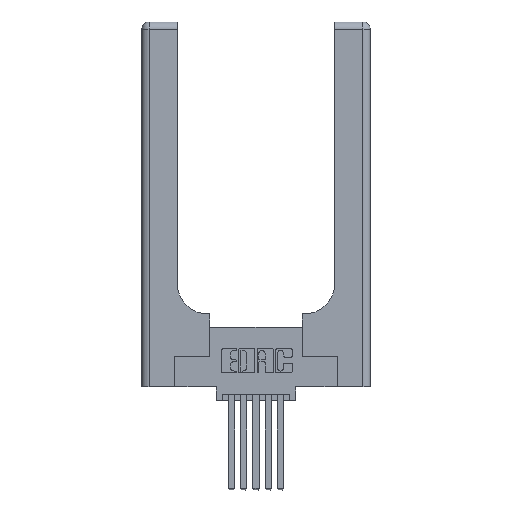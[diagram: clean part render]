
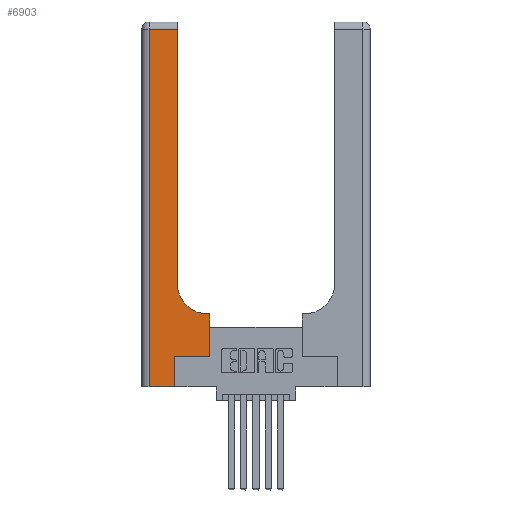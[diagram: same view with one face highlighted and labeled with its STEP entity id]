
A CAD part, top view. The second image highlights one B-rep face of the part: STEP entity #6903.
In plain terms, the highlighted planar face has unit normal (0, 0, 1).
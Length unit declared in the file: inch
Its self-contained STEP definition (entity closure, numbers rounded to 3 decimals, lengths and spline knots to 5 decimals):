
#79 = VERTEX_POINT ( 'NONE', #13041 ) ;
#231 = VECTOR ( 'NONE', #11120, 39.37008 ) ;
#462 = VERTEX_POINT ( 'NONE', #11801 ) ;
#568 = CARTESIAN_POINT ( 'NONE',  ( 0.2915, 3., 0.37 ) ) ;
#622 = LINE ( 'NONE', #8475, #11887 ) ;
#912 = DIRECTION ( 'NONE',  ( 0., 1., 0. ) ) ;
#1087 = VERTEX_POINT ( 'NONE', #9280 ) ;
#1621 = CARTESIAN_POINT ( 'NONE',  ( 0.2915, 0.6, 0.37 ) ) ;
#1825 = ORIENTED_EDGE ( 'NONE', *, *, #13421, .T. ) ;
#1846 = CARTESIAN_POINT ( 'NONE',  ( 0.269, 0.25, 0.37 ) ) ;
#1917 = ORIENTED_EDGE ( 'NONE', *, *, #9651, .T. ) ;
#2306 = VECTOR ( 'NONE', #8315, 39.37008 ) ;
#2355 = CARTESIAN_POINT ( 'NONE',  ( 0., 3., 0.37 ) ) ;
#2364 = VERTEX_POINT ( 'NONE', #2557 ) ;
#2557 = CARTESIAN_POINT ( 'NONE',  ( 0.2915, 2.94, 0.37 ) ) ;
#2765 = DIRECTION ( 'NONE',  ( -1., 0., 0. ) ) ;
#2800 = EDGE_CURVE ( 'NONE', #8301, #1087, #9077, .T. ) ;
#2803 = LINE ( 'NONE', #1846, #5424 ) ;
#2892 = ORIENTED_EDGE ( 'NONE', *, *, #10429, .T. ) ;
#2971 = AXIS2_PLACEMENT_3D ( 'NONE', #6559, #13859, #7617 ) ;
#3492 = EDGE_CURVE ( 'NONE', #11928, #79, #4514, .T. ) ;
#3666 = VERTEX_POINT ( 'NONE', #7474 ) ;
#3703 = VERTEX_POINT ( 'NONE', #7651 ) ;
#3852 = EDGE_CURVE ( 'NONE', #2364, #3666, #8396, .T. ) ;
#4004 = CARTESIAN_POINT ( 'NONE',  ( 0.5585, 0.25, 0.37 ) ) ;
#4514 = LINE ( 'NONE', #10444, #10226 ) ;
#5068 = LINE ( 'NONE', #1621, #7611 ) ;
#5331 = VECTOR ( 'NONE', #912, 39.37008 ) ;
#5424 = VECTOR ( 'NONE', #6294, 39.37008 ) ;
#5729 = DIRECTION ( 'NONE',  ( 0., 0., -1. ) ) ;
#6140 = ORIENTED_EDGE ( 'NONE', *, *, #2800, .T. ) ;
#6294 = DIRECTION ( 'NONE',  ( 1., 0., 0. ) ) ;
#6405 = DIRECTION ( 'NONE',  ( 0., -1., 0. ) ) ;
#6559 = CARTESIAN_POINT ( 'NONE',  ( 0.5415, 0.85, 0.37 ) ) ;
#6763 = AXIS2_PLACEMENT_3D ( 'NONE', #2355, #5729, #13114 ) ;
#6903 = ADVANCED_FACE ( 'NONE', ( #11786 ), #12082, .F. ) ;
#7474 = CARTESIAN_POINT ( 'NONE',  ( 0.06, 2.94, 0.37 ) ) ;
#7580 = CARTESIAN_POINT ( 'NONE',  ( 0.269, 0., 0.37 ) ) ;
#7611 = VECTOR ( 'NONE', #2765, 39.37008 ) ;
#7617 = DIRECTION ( 'NONE',  ( 1., 0., 0. ) ) ;
#7651 = CARTESIAN_POINT ( 'NONE',  ( 0.5415, 0.6, 0.37 ) ) ;
#7864 = LINE ( 'NONE', #7580, #5331 ) ;
#8301 = VERTEX_POINT ( 'NONE', #11116 ) ;
#8315 = DIRECTION ( 'NONE',  ( 0., 1., 0. ) ) ;
#8396 = LINE ( 'NONE', #13668, #11205 ) ;
#8404 = CARTESIAN_POINT ( 'NONE',  ( 0.06, 0., 0.37 ) ) ;
#8475 = CARTESIAN_POINT ( 'NONE',  ( 0.06, 3., 0.37 ) ) ;
#8919 = ORIENTED_EDGE ( 'NONE', *, *, #3852, .T. ) ;
#9077 = LINE ( 'NONE', #4004, #231 ) ;
#9280 = CARTESIAN_POINT ( 'NONE',  ( 0.5585, 0.6, 0.37 ) ) ;
#9651 = EDGE_CURVE ( 'NONE', #79, #12232, #7864, .T. ) ;
#10226 = VECTOR ( 'NONE', #10426, 39.37008 ) ;
#10426 = DIRECTION ( 'NONE',  ( 1., 0., 0. ) ) ;
#10429 = EDGE_CURVE ( 'NONE', #3703, #462, #10659, .T. ) ;
#10444 = CARTESIAN_POINT ( 'NONE',  ( 0., 0., 0.37 ) ) ;
#10619 = LINE ( 'NONE', #568, #2306 ) ;
#10659 = CIRCLE ( 'NONE', #2971, 0.25 ) ;
#10823 = ORIENTED_EDGE ( 'NONE', *, *, #12935, .T. ) ;
#11116 = CARTESIAN_POINT ( 'NONE',  ( 0.5585, 0.25, 0.37 ) ) ;
#11120 = DIRECTION ( 'NONE',  ( 0., 1., 0. ) ) ;
#11205 = VECTOR ( 'NONE', #13916, 39.37008 ) ;
#11786 = FACE_OUTER_BOUND ( 'NONE', #13291, .T. ) ;
#11801 = CARTESIAN_POINT ( 'NONE',  ( 0.2915, 0.85, 0.37 ) ) ;
#11870 = EDGE_CURVE ( 'NONE', #462, #2364, #10619, .T. ) ;
#11887 = VECTOR ( 'NONE', #6405, 39.37008 ) ;
#11928 = VERTEX_POINT ( 'NONE', #8404 ) ;
#12004 = CARTESIAN_POINT ( 'NONE',  ( 0.269, 0.25, 0.37 ) ) ;
#12082 = PLANE ( 'NONE',  #6763 ) ;
#12232 = VERTEX_POINT ( 'NONE', #12004 ) ;
#12399 = ORIENTED_EDGE ( 'NONE', *, *, #3492, .T. ) ;
#12679 = ORIENTED_EDGE ( 'NONE', *, *, #11870, .T. ) ;
#12935 = EDGE_CURVE ( 'NONE', #12232, #8301, #2803, .T. ) ;
#13041 = CARTESIAN_POINT ( 'NONE',  ( 0.269, 0., 0.37 ) ) ;
#13114 = DIRECTION ( 'NONE',  ( -1., 0., 0. ) ) ;
#13291 = EDGE_LOOP ( 'NONE', ( #12679, #8919, #13394, #12399, #1917, #10823, #6140, #1825, #2892 ) ) ;
#13394 = ORIENTED_EDGE ( 'NONE', *, *, #13966, .T. ) ;
#13421 = EDGE_CURVE ( 'NONE', #1087, #3703, #5068, .T. ) ;
#13668 = CARTESIAN_POINT ( 'NONE',  ( 0., 2.94, 0.37 ) ) ;
#13859 = DIRECTION ( 'NONE',  ( 0., 0., -1. ) ) ;
#13916 = DIRECTION ( 'NONE',  ( -1., 0., 0. ) ) ;
#13966 = EDGE_CURVE ( 'NONE', #3666, #11928, #622, .T. ) ;
